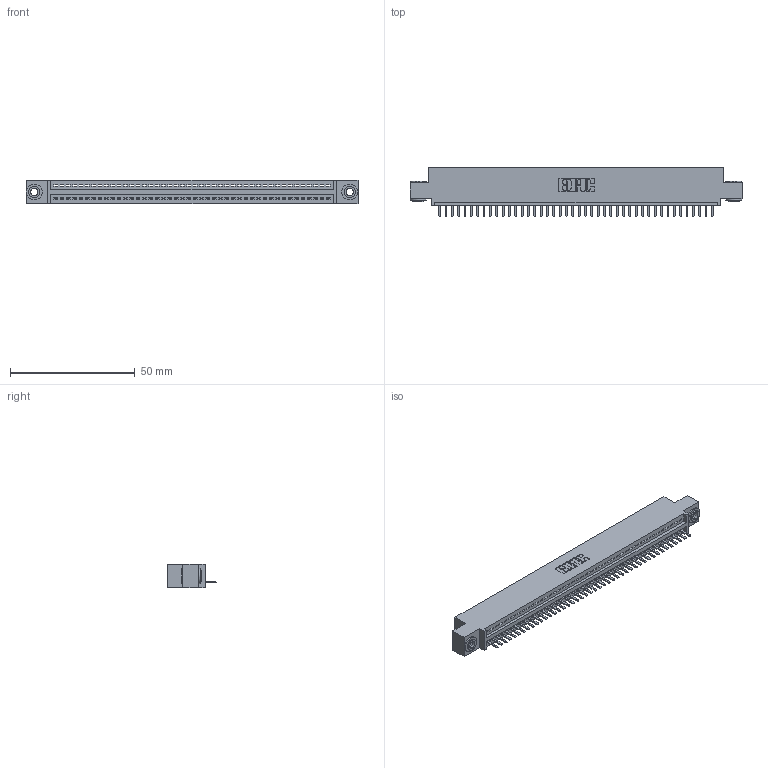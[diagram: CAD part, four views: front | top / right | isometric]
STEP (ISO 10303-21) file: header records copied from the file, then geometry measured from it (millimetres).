
FILE_DESCRIPTION (( 'STEP AP203' ), '1' );
FILE_NAME ('345-044-520-403.STEP', '2018-09-08T09:14:12', ( '' ), ( '' ), 'SwSTEP 2.0', 'SolidWorks 2016', '' );
FILE_SCHEMA (( 'CONFIG_CONTROL_DESIGN' ));
Length unit declared in the file: inch
Products named in the file (4): 345 Part_0.110 Offset - 0.156 Dia-TH; 345-292-001_345-293-120; 345-250-002_345-250-002-102; 345-044-520-403
Assembly tree (47 placements, depth 2):
  345-044-520-403
    345 Part_0.110 Offset - 0.156 Dia-TH
    345-292-001_345-293-120  x44
    345-250-002_345-250-002-102  x2
Bounding box: 132.97 x 19.68 x 9.4 mm (x, y, z)
Volume: 12465.4 mm3; surface area: 16474.8 mm2
Topology: 47 solids, 47 shells, 2896 faces, 8525 edges, 5562 vertices
Faces by surface type: plane 1942, cylinder 946, cone 8
Entity records: 33742 total; most frequent: CARTESIAN_POINT 5835, ORIENTED_EDGE 5794, DIRECTION 5111, EDGE_CURVE 2897, LINE 2561, VECTOR 2561, VERTEX_POINT 1926, AXIS2_PLACEMENT_3D 1275
